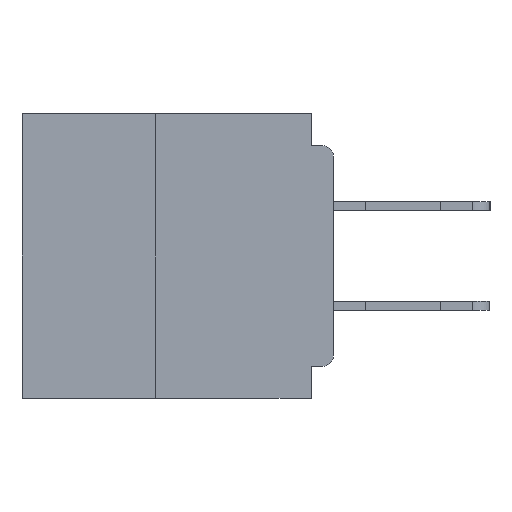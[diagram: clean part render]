
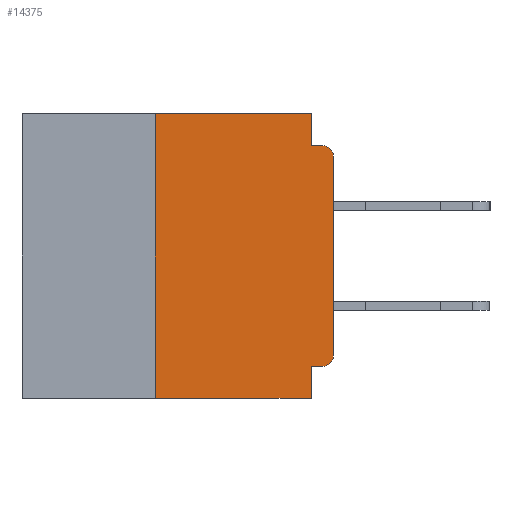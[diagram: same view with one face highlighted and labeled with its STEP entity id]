
A CAD part, left-side view. The second image highlights one B-rep face of the part: STEP entity #14375.
In plain terms, the highlighted planar face has unit normal (-1, 0, 0).
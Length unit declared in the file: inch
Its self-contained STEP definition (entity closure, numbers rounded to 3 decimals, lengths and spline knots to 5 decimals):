
#61 = CARTESIAN_POINT ( 'NONE',  ( 0., 0., -0.06 ) ) ;
#275 = VECTOR ( 'NONE', #32521, 39.37008 ) ;
#529 = DIRECTION ( 'NONE',  ( 0., -1., 0. ) ) ;
#1518 = VERTEX_POINT ( 'NONE', #29432 ) ;
#1609 = LINE ( 'NONE', #42520, #26313 ) ;
#3133 = VERTEX_POINT ( 'NONE', #25799 ) ;
#4623 = VERTEX_POINT ( 'NONE', #36892 ) ;
#5023 = CARTESIAN_POINT ( 'NONE',  ( 0., 0.015, -0.06 ) ) ;
#5041 = CARTESIAN_POINT ( 'NONE',  ( 0., 0., -0.34 ) ) ;
#7006 = DIRECTION ( 'NONE',  ( 1., 0., 0. ) ) ;
#7652 = ORIENTED_EDGE ( 'NONE', *, *, #17876, .F. ) ;
#8432 = DIRECTION ( 'NONE',  ( 0., 0., -1. ) ) ;
#9512 = ORIENTED_EDGE ( 'NONE', *, *, #15453, .T. ) ;
#10521 = LINE ( 'NONE', #29602, #36045 ) ;
#10613 = ORIENTED_EDGE ( 'NONE', *, *, #13552, .F. ) ;
#10868 = DIRECTION ( 'NONE',  ( 0., -1., 0. ) ) ;
#11913 = ORIENTED_EDGE ( 'NONE', *, *, #31487, .F. ) ;
#12509 = CARTESIAN_POINT ( 'NONE',  ( 0., 0.25, -0.4 ) ) ;
#13552 = EDGE_CURVE ( 'NONE', #24576, #17379, #31816, .T. ) ;
#14375 = ADVANCED_FACE ( 'NONE', ( #34846 ), #40216, .F. ) ;
#14458 = DIRECTION ( 'NONE',  ( -1., 0., 0. ) ) ;
#15308 = CARTESIAN_POINT ( 'NONE',  ( 0., 0.031, -0.355 ) ) ;
#15453 = EDGE_CURVE ( 'NONE', #35105, #37134, #40878, .T. ) ;
#15573 = EDGE_CURVE ( 'NONE', #1518, #33035, #35709, .T. ) ;
#15790 = EDGE_CURVE ( 'NONE', #17379, #3133, #28467, .T. ) ;
#16571 = ORIENTED_EDGE ( 'NONE', *, *, #15573, .F. ) ;
#16822 = AXIS2_PLACEMENT_3D ( 'NONE', #5023, #28480, #8432 ) ;
#16833 = VERTEX_POINT ( 'NONE', #22669 ) ;
#17379 = VERTEX_POINT ( 'NONE', #38865 ) ;
#17487 = VECTOR ( 'NONE', #529, 39.37008 ) ;
#17876 = EDGE_CURVE ( 'NONE', #33035, #4623, #10521, .T. ) ;
#18967 = CARTESIAN_POINT ( 'NONE',  ( 0., 0., -0.355 ) ) ;
#19729 = AXIS2_PLACEMENT_3D ( 'NONE', #23722, #7006, #30443 ) ;
#20540 = ORIENTED_EDGE ( 'NONE', *, *, #20752, .T. ) ;
#20752 = EDGE_CURVE ( 'NONE', #38236, #35105, #25997, .T. ) ;
#21043 = ORIENTED_EDGE ( 'NONE', *, *, #15790, .F. ) ;
#21104 = DIRECTION ( 'NONE',  ( 0., 0., 1. ) ) ;
#22300 = DIRECTION ( 'NONE',  ( 0., -1., 0. ) ) ;
#22313 = DIRECTION ( 'NONE',  ( 0., 1., 0. ) ) ;
#22661 = ORIENTED_EDGE ( 'NONE', *, *, #39568, .F. ) ;
#22669 = CARTESIAN_POINT ( 'NONE',  ( 0., 0.031, -0.045 ) ) ;
#23722 = CARTESIAN_POINT ( 'NONE',  ( 0., 0.437, 0. ) ) ;
#24576 = VERTEX_POINT ( 'NONE', #41710 ) ;
#25762 = LINE ( 'NONE', #38841, #26801 ) ;
#25799 = CARTESIAN_POINT ( 'NONE',  ( 0., 0.031, 0. ) ) ;
#25997 = LINE ( 'NONE', #37658, #42547 ) ;
#26043 = DIRECTION ( 'NONE',  ( 0., 0., -1. ) ) ;
#26313 = VECTOR ( 'NONE', #26043, 39.37008 ) ;
#26801 = VECTOR ( 'NONE', #22300, 39.37008 ) ;
#26884 = VECTOR ( 'NONE', #22313, 39.37008 ) ;
#27149 = EDGE_CURVE ( 'NONE', #1518, #38236, #38226, .T. ) ;
#27519 = AXIS2_PLACEMENT_3D ( 'NONE', #34416, #14458, #37728 ) ;
#27523 = CARTESIAN_POINT ( 'NONE',  ( 0., 0.437, -0.4 ) ) ;
#28294 = CARTESIAN_POINT ( 'NONE',  ( 0., 0.015, -0.045 ) ) ;
#28467 = LINE ( 'NONE', #40573, #17487 ) ;
#28480 = DIRECTION ( 'NONE',  ( -1., 0., 0. ) ) ;
#29432 = CARTESIAN_POINT ( 'NONE',  ( 0., 0.015, -0.355 ) ) ;
#29602 = CARTESIAN_POINT ( 'NONE',  ( 0., 0.031, -0.4 ) ) ;
#30378 = VECTOR ( 'NONE', #10868, 39.37008 ) ;
#30443 = DIRECTION ( 'NONE',  ( 0., 0., -1. ) ) ;
#31487 = EDGE_CURVE ( 'NONE', #16833, #37134, #25762, .T. ) ;
#31816 = LINE ( 'NONE', #12509, #275 ) ;
#32466 = LINE ( 'NONE', #27523, #30378 ) ;
#32521 = DIRECTION ( 'NONE',  ( 0., 0., 1. ) ) ;
#33035 = VERTEX_POINT ( 'NONE', #15308 ) ;
#34416 = CARTESIAN_POINT ( 'NONE',  ( 0., 0.015, -0.34 ) ) ;
#34665 = EDGE_LOOP ( 'NONE', ( #20540, #9512, #11913, #22661, #21043, #10613, #34995, #7652, #16571, #36033 ) ) ;
#34846 = FACE_OUTER_BOUND ( 'NONE', #34665, .T. ) ;
#34995 = ORIENTED_EDGE ( 'NONE', *, *, #41499, .T. ) ;
#35105 = VERTEX_POINT ( 'NONE', #61 ) ;
#35709 = LINE ( 'NONE', #18967, #26884 ) ;
#36033 = ORIENTED_EDGE ( 'NONE', *, *, #27149, .T. ) ;
#36045 = VECTOR ( 'NONE', #39542, 39.37008 ) ;
#36892 = CARTESIAN_POINT ( 'NONE',  ( 0., 0.031, -0.4 ) ) ;
#37134 = VERTEX_POINT ( 'NONE', #28294 ) ;
#37658 = CARTESIAN_POINT ( 'NONE',  ( 0., 0., 0. ) ) ;
#37728 = DIRECTION ( 'NONE',  ( 0., 0., -1. ) ) ;
#38226 = CIRCLE ( 'NONE', #27519, 0.015 ) ;
#38236 = VERTEX_POINT ( 'NONE', #5041 ) ;
#38841 = CARTESIAN_POINT ( 'NONE',  ( 0., 0., -0.045 ) ) ;
#38865 = CARTESIAN_POINT ( 'NONE',  ( 0., 0.25, 0. ) ) ;
#39542 = DIRECTION ( 'NONE',  ( 0., 0., -1. ) ) ;
#39568 = EDGE_CURVE ( 'NONE', #3133, #16833, #1609, .T. ) ;
#40216 = PLANE ( 'NONE',  #19729 ) ;
#40573 = CARTESIAN_POINT ( 'NONE',  ( 0., 0.437, 0. ) ) ;
#40878 = CIRCLE ( 'NONE', #16822, 0.015 ) ;
#41499 = EDGE_CURVE ( 'NONE', #24576, #4623, #32466, .T. ) ;
#41710 = CARTESIAN_POINT ( 'NONE',  ( 0., 0.25, -0.4 ) ) ;
#42520 = CARTESIAN_POINT ( 'NONE',  ( 0., 0.031, 0. ) ) ;
#42547 = VECTOR ( 'NONE', #21104, 39.37008 ) ;
